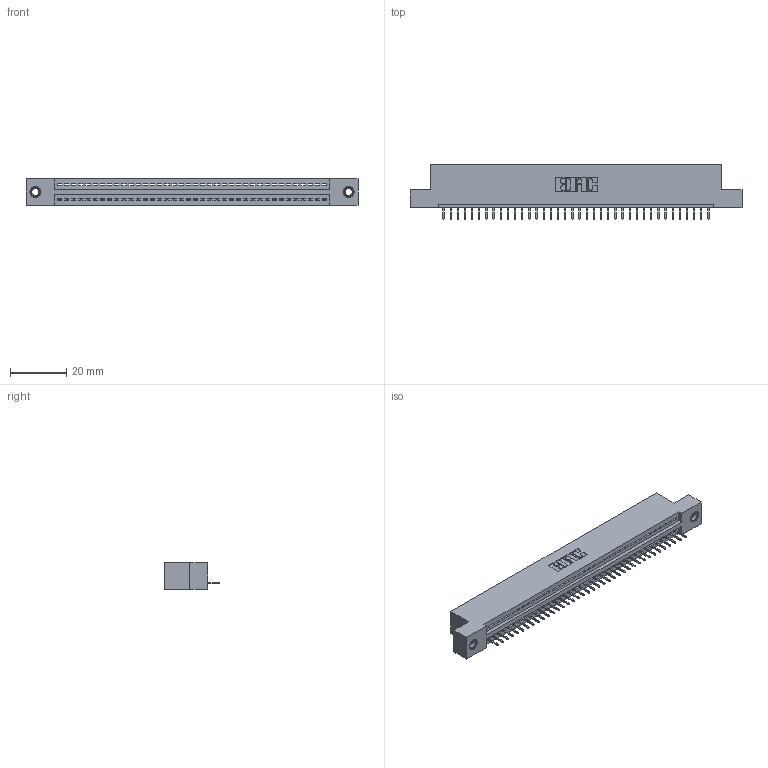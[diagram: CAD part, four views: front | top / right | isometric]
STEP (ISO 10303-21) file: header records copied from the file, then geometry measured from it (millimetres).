
FILE_DESCRIPTION (( 'STEP AP203' ), '1' );
FILE_NAME ('395-038-524-107.STEP', '2019-10-22T00:59:16', ( '' ), ( '' ), 'SwSTEP 2.0', 'SolidWorks 2016', '' );
FILE_SCHEMA (( 'CONFIG_CONTROL_DESIGN' ));
Length unit declared in the file: inch
Products named in the file (4): 395-038-524-107; 345-292-001_345-293-124; 345 Part_Flush Mounting Lugs - 0.156 Dia-TI; 345-250-001_345-250-005-103
Assembly tree (41 placements, depth 2):
  395-038-524-107
    345 Part_Flush Mounting Lugs - 0.156 Dia-TI
    345-292-001_345-293-124  x38
    345-250-001_345-250-005-103  x2
Bounding box: 117.73 x 19.35 x 9.4 mm (x, y, z)
Volume: 10985.6 mm3; surface area: 14097.1 mm2
Topology: 41 solids, 41 shells, 2542 faces, 7317 edges, 4718 vertices
Faces by surface type: plane 1860, cylinder 666, cone 12, torus 4
Entity records: 30398 total; most frequent: CARTESIAN_POINT 5245, ORIENTED_EDGE 5210, DIRECTION 4615, EDGE_CURVE 2605, LINE 2305, VECTOR 2305, VERTEX_POINT 1728, AXIS2_PLACEMENT_3D 1155
